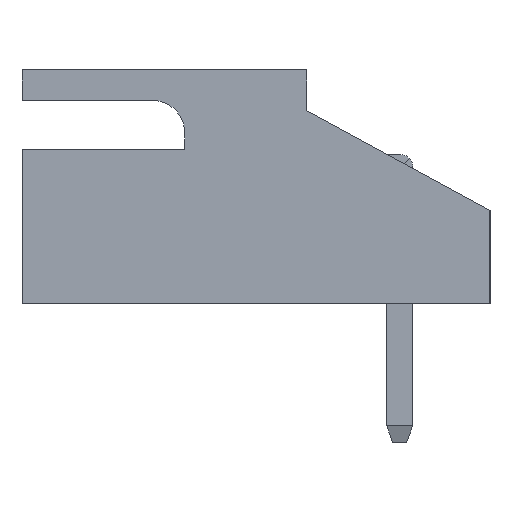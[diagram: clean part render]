
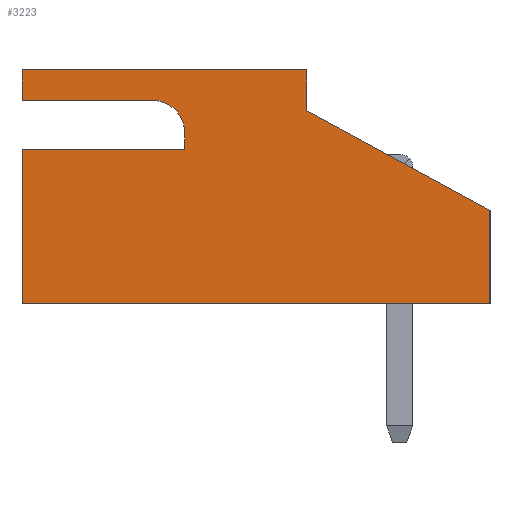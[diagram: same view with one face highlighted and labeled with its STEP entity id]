
A CAD part, left-side view. The second image highlights one B-rep face of the part: STEP entity #3223.
In plain terms, the highlighted planar face has unit normal (-1, 0, 0).
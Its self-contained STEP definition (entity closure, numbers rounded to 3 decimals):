
#4 = CARTESIAN_POINT ( 'NONE',  ( -8.75, 3.8, 1.325 ) ) ;
#78 = VERTEX_POINT ( 'NONE', #2999 ) ;
#114 = VECTOR ( 'NONE', #2382, 1000. ) ;
#130 = VECTOR ( 'NONE', #581, 1000. ) ;
#182 = LINE ( 'NONE', #2230, #199 ) ;
#199 = VECTOR ( 'NONE', #2919, 1000. ) ;
#281 = LINE ( 'NONE', #1714, #114 ) ;
#285 = DIRECTION ( 'NONE',  ( 0., -1., 0. ) ) ;
#410 = VECTOR ( 'NONE', #4137, 1000. ) ;
#519 = ORIENTED_EDGE ( 'NONE', *, *, #3734, .T. ) ;
#581 = DIRECTION ( 'NONE',  ( 0., 0., 1. ) ) ;
#712 = CARTESIAN_POINT ( 'NONE',  ( -8.75, 0., 1.875 ) ) ;
#727 = VECTOR ( 'NONE', #1449, 1000. ) ;
#809 = VERTEX_POINT ( 'NONE', #1466 ) ;
#847 = LINE ( 'NONE', #1147, #3010 ) ;
#858 = LINE ( 'NONE', #1566, #410 ) ;
#891 = DIRECTION ( 'NONE',  ( 1., 0., 0. ) ) ;
#904 = EDGE_CURVE ( 'NONE', #2838, #1638, #847, .T. ) ;
#939 = AXIS2_PLACEMENT_3D ( 'NONE', #4, #2845, #2483 ) ;
#976 = CARTESIAN_POINT ( 'NONE',  ( -8.75, 3., 0.925 ) ) ;
#1035 = VERTEX_POINT ( 'NONE', #3761 ) ;
#1087 = VERTEX_POINT ( 'NONE', #976 ) ;
#1147 = CARTESIAN_POINT ( 'NONE',  ( -8.75, -4.5, -0.575 ) ) ;
#1271 = VERTEX_POINT ( 'NONE', #3524 ) ;
#1350 = ORIENTED_EDGE ( 'NONE', *, *, #2673, .F. ) ;
#1449 = DIRECTION ( 'NONE',  ( 0., -0.878, -0.478 ) ) ;
#1466 = CARTESIAN_POINT ( 'NONE',  ( -8.75, 7., 0.925 ) ) ;
#1483 = CARTESIAN_POINT ( 'NONE',  ( -8.75, 7., -2.875 ) ) ;
#1520 = DIRECTION ( 'NONE',  ( 0., -1., 0. ) ) ;
#1566 = CARTESIAN_POINT ( 'NONE',  ( -8.75, 7., 2.125 ) ) ;
#1592 = VECTOR ( 'NONE', #2740, 1000. ) ;
#1638 = VERTEX_POINT ( 'NONE', #2433 ) ;
#1641 = CARTESIAN_POINT ( 'NONE',  ( -8.75, 7., 2.125 ) ) ;
#1700 = CARTESIAN_POINT ( 'NONE',  ( -8.75, 7., 2.875 ) ) ;
#1714 = CARTESIAN_POINT ( 'NONE',  ( -8.75, 0., -2.875 ) ) ;
#1848 = ORIENTED_EDGE ( 'NONE', *, *, #3284, .T. ) ;
#2073 = ORIENTED_EDGE ( 'NONE', *, *, #3539, .T. ) ;
#2114 = EDGE_CURVE ( 'NONE', #3051, #809, #3104, .T. ) ;
#2230 = CARTESIAN_POINT ( 'NONE',  ( -8.75, 3., 1.325 ) ) ;
#2246 = CARTESIAN_POINT ( 'NONE',  ( -8.75, 7., -2.875 ) ) ;
#2382 = DIRECTION ( 'NONE',  ( 0., 0., 1. ) ) ;
#2433 = CARTESIAN_POINT ( 'NONE',  ( -8.75, -4.5, -2.875 ) ) ;
#2445 = VERTEX_POINT ( 'NONE', #2452 ) ;
#2452 = CARTESIAN_POINT ( 'NONE',  ( -8.75, 3.8, 2.125 ) ) ;
#2483 = DIRECTION ( 'NONE',  ( 0., 0., -1. ) ) ;
#2514 = EDGE_CURVE ( 'NONE', #1087, #809, #4485, .T. ) ;
#2521 = ORIENTED_EDGE ( 'NONE', *, *, #2961, .F. ) ;
#2525 = VERTEX_POINT ( 'NONE', #4159 ) ;
#2541 = LINE ( 'NONE', #712, #727 ) ;
#2620 = DIRECTION ( 'NONE',  ( 0., 0., 1. ) ) ;
#2673 = EDGE_CURVE ( 'NONE', #3380, #2525, #3183, .T. ) ;
#2740 = DIRECTION ( 'NONE',  ( 0., 1., 0. ) ) ;
#2760 = ORIENTED_EDGE ( 'NONE', *, *, #2514, .T. ) ;
#2784 = AXIS2_PLACEMENT_3D ( 'NONE', #3646, #891, #3666 ) ;
#2829 = CARTESIAN_POINT ( 'NONE',  ( -8.75, 7., -2.875 ) ) ;
#2838 = VERTEX_POINT ( 'NONE', #3417 ) ;
#2845 = DIRECTION ( 'NONE',  ( 1., 0., 0. ) ) ;
#2848 = ORIENTED_EDGE ( 'NONE', *, *, #3214, .T. ) ;
#2919 = DIRECTION ( 'NONE',  ( 0., 0., -1. ) ) ;
#2950 = DIRECTION ( 'NONE',  ( 0., 0., -1. ) ) ;
#2961 = EDGE_CURVE ( 'NONE', #2525, #78, #3805, .T. ) ;
#2991 = EDGE_CURVE ( 'NONE', #2445, #1271, #3904, .T. ) ;
#2999 = CARTESIAN_POINT ( 'NONE',  ( -8.75, 0., 2.875 ) ) ;
#3010 = VECTOR ( 'NONE', #2950, 1000. ) ;
#3051 = VERTEX_POINT ( 'NONE', #1483 ) ;
#3104 = LINE ( 'NONE', #3751, #130 ) ;
#3146 = EDGE_LOOP ( 'NONE', ( #1350, #2073, #3362, #2848, #2760, #3905, #519, #4395, #4053, #1848, #2521 ) ) ;
#3183 = LINE ( 'NONE', #2829, #4420 ) ;
#3214 = EDGE_CURVE ( 'NONE', #1271, #1087, #182, .T. ) ;
#3223 = ADVANCED_FACE ( 'NONE', ( #4060 ), #4344, .F. ) ;
#3284 = EDGE_CURVE ( 'NONE', #1035, #78, #281, .T. ) ;
#3362 = ORIENTED_EDGE ( 'NONE', *, *, #2991, .T. ) ;
#3380 = VERTEX_POINT ( 'NONE', #1641 ) ;
#3417 = CARTESIAN_POINT ( 'NONE',  ( -8.75, -4.5, -0.575 ) ) ;
#3444 = CARTESIAN_POINT ( 'NONE',  ( -8.75, 7., 0.925 ) ) ;
#3524 = CARTESIAN_POINT ( 'NONE',  ( -8.75, 3., 1.325 ) ) ;
#3539 = EDGE_CURVE ( 'NONE', #3380, #2445, #858, .T. ) ;
#3646 = CARTESIAN_POINT ( 'NONE',  ( -8.75, 7., -2.875 ) ) ;
#3666 = DIRECTION ( 'NONE',  ( 0., 0., -1. ) ) ;
#3734 = EDGE_CURVE ( 'NONE', #3051, #1638, #4389, .T. ) ;
#3751 = CARTESIAN_POINT ( 'NONE',  ( -8.75, 7., -2.875 ) ) ;
#3761 = CARTESIAN_POINT ( 'NONE',  ( -8.75, 0., 1.875 ) ) ;
#3805 = LINE ( 'NONE', #1700, #4278 ) ;
#3904 = CIRCLE ( 'NONE', #939, 0.8 ) ;
#3905 = ORIENTED_EDGE ( 'NONE', *, *, #2114, .F. ) ;
#3971 = VECTOR ( 'NONE', #1520, 1000. ) ;
#4053 = ORIENTED_EDGE ( 'NONE', *, *, #4097, .F. ) ;
#4060 = FACE_OUTER_BOUND ( 'NONE', #3146, .T. ) ;
#4097 = EDGE_CURVE ( 'NONE', #1035, #2838, #2541, .T. ) ;
#4137 = DIRECTION ( 'NONE',  ( 0., -1., 0. ) ) ;
#4159 = CARTESIAN_POINT ( 'NONE',  ( -8.75, 7., 2.875 ) ) ;
#4278 = VECTOR ( 'NONE', #285, 1000. ) ;
#4344 = PLANE ( 'NONE',  #2784 ) ;
#4389 = LINE ( 'NONE', #2246, #3971 ) ;
#4395 = ORIENTED_EDGE ( 'NONE', *, *, #904, .F. ) ;
#4420 = VECTOR ( 'NONE', #2620, 1000. ) ;
#4485 = LINE ( 'NONE', #3444, #1592 ) ;
